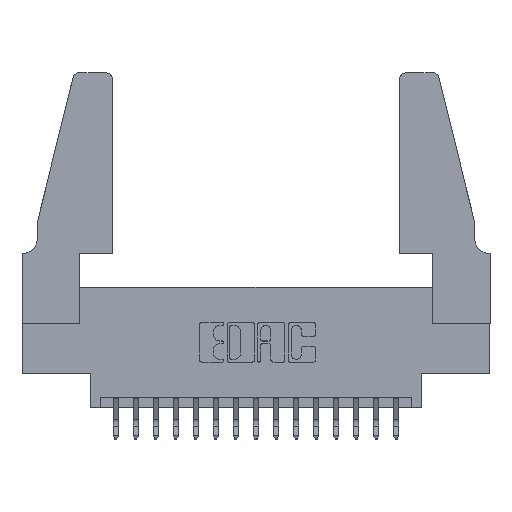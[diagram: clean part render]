
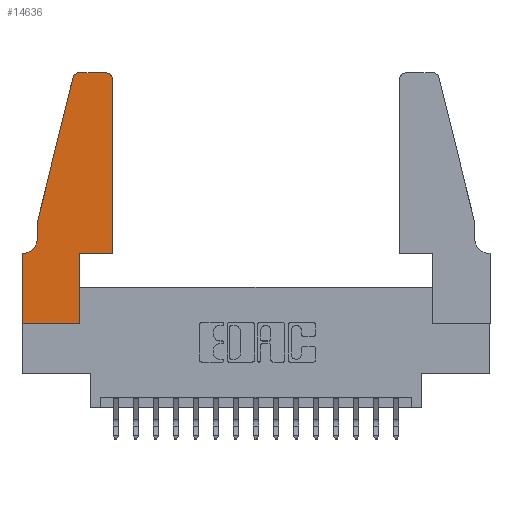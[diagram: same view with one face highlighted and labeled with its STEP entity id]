
A CAD part, top view. The second image highlights one B-rep face of the part: STEP entity #14636.
In plain terms, the highlighted planar face has unit normal (0, 0, 1).
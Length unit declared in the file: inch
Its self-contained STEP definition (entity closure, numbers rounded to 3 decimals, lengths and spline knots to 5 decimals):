
#63 = VERTEX_POINT ( 'NONE', #6341 ) ;
#198 = DIRECTION ( 'NONE',  ( 0., 0., 1. ) ) ;
#239 = VECTOR ( 'NONE', #2415, 39.37008 ) ;
#602 = DIRECTION ( 'NONE',  ( 0., -1., 0. ) ) ;
#700 = ORIENTED_EDGE ( 'NONE', *, *, #2888, .T. ) ;
#711 = LINE ( 'NONE', #7738, #7797 ) ;
#838 = ORIENTED_EDGE ( 'NONE', *, *, #14503, .T. ) ;
#1088 = LINE ( 'NONE', #9808, #11760 ) ;
#1186 = CARTESIAN_POINT ( 'NONE',  ( 0.4505, 0.35, 0.37 ) ) ;
#1188 = ORIENTED_EDGE ( 'NONE', *, *, #12583, .T. ) ;
#1237 = CARTESIAN_POINT ( 'NONE',  ( 0.284, 1.22, 0.37 ) ) ;
#1267 = VECTOR ( 'NONE', #8875, 39.37008 ) ;
#1444 = VECTOR ( 'NONE', #17866, 39.37008 ) ;
#1850 = PLANE ( 'NONE',  #16281 ) ;
#1971 = CARTESIAN_POINT ( 'NONE',  ( 0.0755, 0.42, 0.37 ) ) ;
#2086 = CARTESIAN_POINT ( 'NONE',  ( 0.0055, 0.42, 0.37 ) ) ;
#2215 = CARTESIAN_POINT ( 'NONE',  ( 0., 0., 0.37 ) ) ;
#2244 = VERTEX_POINT ( 'NONE', #3733 ) ;
#2298 = EDGE_CURVE ( 'NONE', #4224, #2822, #6302, .T. ) ;
#2415 = DIRECTION ( 'NONE',  ( 1., 0., 0. ) ) ;
#2781 = ORIENTED_EDGE ( 'NONE', *, *, #3384, .T. ) ;
#2822 = VERTEX_POINT ( 'NONE', #3670 ) ;
#2854 = CIRCLE ( 'NONE', #6133, 0.07 ) ;
#2888 = EDGE_CURVE ( 'NONE', #10319, #4357, #711, .T. ) ;
#3124 = EDGE_CURVE ( 'NONE', #8382, #2244, #8000, .T. ) ;
#3285 = CARTESIAN_POINT ( 'NONE',  ( 0.0755, 0.35, 0.37 ) ) ;
#3344 = EDGE_CURVE ( 'NONE', #2822, #5412, #4040, .T. ) ;
#3384 = EDGE_CURVE ( 'NONE', #4357, #12073, #7783, .T. ) ;
#3486 = DIRECTION ( 'NONE',  ( -1., 0., 0. ) ) ;
#3670 = CARTESIAN_POINT ( 'NONE',  ( 0., 0., 0.37 ) ) ;
#3733 = CARTESIAN_POINT ( 'NONE',  ( 0.4505, 0.35, 0.37 ) ) ;
#4040 = LINE ( 'NONE', #2215, #239 ) ;
#4224 = VERTEX_POINT ( 'NONE', #13497 ) ;
#4357 = VERTEX_POINT ( 'NONE', #17836 ) ;
#4585 = LINE ( 'NONE', #3285, #1267 ) ;
#4756 = DIRECTION ( 'NONE',  ( 1., 0., 0. ) ) ;
#4812 = CARTESIAN_POINT ( 'NONE',  ( 0.0755, 0.5, 0.37 ) ) ;
#5118 = EDGE_CURVE ( 'NONE', #5412, #8382, #1088, .T. ) ;
#5220 = LINE ( 'NONE', #8360, #1444 ) ;
#5394 = EDGE_CURVE ( 'NONE', #12073, #63, #14367, .T. ) ;
#5412 = VERTEX_POINT ( 'NONE', #10399 ) ;
#5563 = CARTESIAN_POINT ( 'NONE',  ( 0.0055, 0.35, 0.37 ) ) ;
#5660 = DIRECTION ( 'NONE',  ( 0., 1., 0. ) ) ;
#6130 = CARTESIAN_POINT ( 'NONE',  ( 0., 0.35, 0.37 ) ) ;
#6133 = AXIS2_PLACEMENT_3D ( 'NONE', #2086, #11785, #3486 ) ;
#6302 = LINE ( 'NONE', #10086, #16809 ) ;
#6341 = CARTESIAN_POINT ( 'NONE',  ( 0.0755, 0.5, 0.37 ) ) ;
#6410 = DIRECTION ( 'NONE',  ( 0., 0., 1. ) ) ;
#6469 = DIRECTION ( 'NONE',  ( 1., 0., 0. ) ) ;
#7738 = CARTESIAN_POINT ( 'NONE',  ( 0.2605, 1.25, 0.37 ) ) ;
#7783 = CIRCLE ( 'NONE', #16634, 0.03 ) ;
#7797 = VECTOR ( 'NONE', #7829, 39.37008 ) ;
#7829 = DIRECTION ( 'NONE',  ( -1., 0., 0. ) ) ;
#7910 = VECTOR ( 'NONE', #14483, 39.37008 ) ;
#7949 = DIRECTION ( 'NONE',  ( 1., 0., 0. ) ) ;
#7996 = CARTESIAN_POINT ( 'NONE',  ( 0.4505, 0.35, 0.37 ) ) ;
#8000 = LINE ( 'NONE', #7996, #10773 ) ;
#8360 = CARTESIAN_POINT ( 'NONE',  ( 0.0755, 0.5, 0.37 ) ) ;
#8382 = VERTEX_POINT ( 'NONE', #9909 ) ;
#8665 = CARTESIAN_POINT ( 'NONE',  ( 0.4205, 1.22, 0.37 ) ) ;
#8817 = VERTEX_POINT ( 'NONE', #5563 ) ;
#8875 = DIRECTION ( 'NONE',  ( -1., 0., 0. ) ) ;
#8963 = ORIENTED_EDGE ( 'NONE', *, *, #3344, .T. ) ;
#9423 = CARTESIAN_POINT ( 'NONE',  ( 0.25487, 1.22718, 0.37 ) ) ;
#9635 = EDGE_CURVE ( 'NONE', #10682, #10319, #12980, .T. ) ;
#9808 = CARTESIAN_POINT ( 'NONE',  ( 0.2865, 0.35, 0.37 ) ) ;
#9909 = CARTESIAN_POINT ( 'NONE',  ( 0.2865, 0.35, 0.37 ) ) ;
#10044 = DIRECTION ( 'NONE',  ( 1., 0., 0. ) ) ;
#10086 = CARTESIAN_POINT ( 'NONE',  ( 0., 0., 0.37 ) ) ;
#10319 = VERTEX_POINT ( 'NONE', #17679 ) ;
#10399 = CARTESIAN_POINT ( 'NONE',  ( 0.2865, 0., 0.37 ) ) ;
#10497 = ORIENTED_EDGE ( 'NONE', *, *, #5118, .T. ) ;
#10503 = ORIENTED_EDGE ( 'NONE', *, *, #15671, .T. ) ;
#10601 = EDGE_LOOP ( 'NONE', ( #700, #2781, #13129, #838, #1188, #14956, #16037, #8963, #10497, #14961, #10503, #13353 ) ) ;
#10682 = VERTEX_POINT ( 'NONE', #14522 ) ;
#10773 = VECTOR ( 'NONE', #7949, 39.37008 ) ;
#11760 = VECTOR ( 'NONE', #5660, 39.37008 ) ;
#11785 = DIRECTION ( 'NONE',  ( 0., 0., -1. ) ) ;
#11971 = VERTEX_POINT ( 'NONE', #1971 ) ;
#12073 = VERTEX_POINT ( 'NONE', #9423 ) ;
#12320 = DIRECTION ( 'NONE',  ( 0., 1., 0. ) ) ;
#12583 = EDGE_CURVE ( 'NONE', #11971, #8817, #2854, .T. ) ;
#12980 = CIRCLE ( 'NONE', #15101, 0.03 ) ;
#13019 = DIRECTION ( 'NONE',  ( 0., 0., 1. ) ) ;
#13129 = ORIENTED_EDGE ( 'NONE', *, *, #5394, .T. ) ;
#13353 = ORIENTED_EDGE ( 'NONE', *, *, #9635, .T. ) ;
#13423 = EDGE_CURVE ( 'NONE', #8817, #4224, #4585, .T. ) ;
#13497 = CARTESIAN_POINT ( 'NONE',  ( 0., 0.35, 0.37 ) ) ;
#14367 = LINE ( 'NONE', #4812, #7910 ) ;
#14483 = DIRECTION ( 'NONE',  ( -0.239, -0.971, 0. ) ) ;
#14503 = EDGE_CURVE ( 'NONE', #63, #11971, #5220, .T. ) ;
#14522 = CARTESIAN_POINT ( 'NONE',  ( 0.4505, 1.22, 0.37 ) ) ;
#14636 = ADVANCED_FACE ( 'NONE', ( #16825 ), #1850, .T. ) ;
#14956 = ORIENTED_EDGE ( 'NONE', *, *, #13423, .T. ) ;
#14961 = ORIENTED_EDGE ( 'NONE', *, *, #3124, .T. ) ;
#15101 = AXIS2_PLACEMENT_3D ( 'NONE', #8665, #198, #10044 ) ;
#15118 = LINE ( 'NONE', #1186, #15546 ) ;
#15546 = VECTOR ( 'NONE', #12320, 39.37008 ) ;
#15671 = EDGE_CURVE ( 'NONE', #2244, #10682, #15118, .T. ) ;
#16037 = ORIENTED_EDGE ( 'NONE', *, *, #2298, .T. ) ;
#16281 = AXIS2_PLACEMENT_3D ( 'NONE', #6130, #13019, #4756 ) ;
#16634 = AXIS2_PLACEMENT_3D ( 'NONE', #1237, #6410, #6469 ) ;
#16809 = VECTOR ( 'NONE', #602, 39.37008 ) ;
#16825 = FACE_OUTER_BOUND ( 'NONE', #10601, .T. ) ;
#17679 = CARTESIAN_POINT ( 'NONE',  ( 0.4205, 1.25, 0.37 ) ) ;
#17836 = CARTESIAN_POINT ( 'NONE',  ( 0.284, 1.25, 0.37 ) ) ;
#17866 = DIRECTION ( 'NONE',  ( 0., -1., 0. ) ) ;
